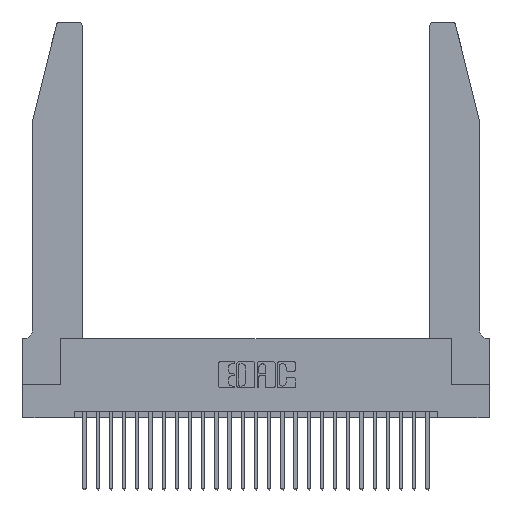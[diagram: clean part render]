
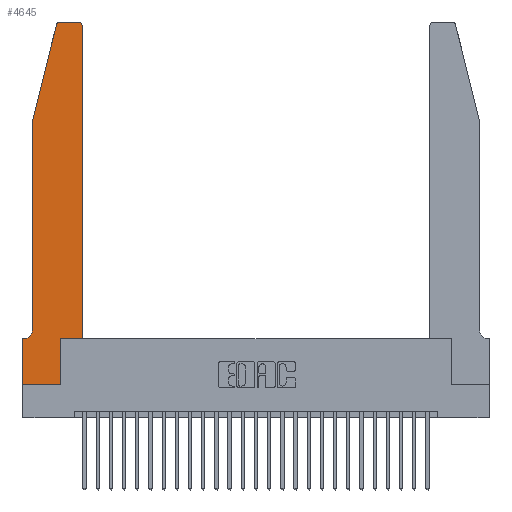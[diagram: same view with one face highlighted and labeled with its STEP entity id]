
A CAD part, top view. The second image highlights one B-rep face of the part: STEP entity #4645.
In plain terms, the highlighted planar face has unit normal (0, 0, 1).
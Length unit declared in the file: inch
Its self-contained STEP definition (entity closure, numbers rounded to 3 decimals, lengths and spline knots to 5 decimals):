
#270 = DIRECTION ( 'NONE',  ( 1., 0., 0. ) ) ;
#932 = DIRECTION ( 'NONE',  ( 1., 0., 0. ) ) ;
#1057 = DIRECTION ( 'NONE',  ( 0., -1., 0. ) ) ;
#1145 = ORIENTED_EDGE ( 'NONE', *, *, #22126, .T. ) ;
#1323 = DIRECTION ( 'NONE',  ( 0., 0., -1. ) ) ;
#1381 = CARTESIAN_POINT ( 'NONE',  ( 0., 0., 0.37 ) ) ;
#1448 = CARTESIAN_POINT ( 'NONE',  ( 0.2605, 2.75, 0.37 ) ) ;
#2068 = VERTEX_POINT ( 'NONE', #8273 ) ;
#2185 = CIRCLE ( 'NONE', #24513, 0.07 ) ;
#3472 = CARTESIAN_POINT ( 'NONE',  ( 0.2865, 0.35, 0.37 ) ) ;
#3636 = EDGE_CURVE ( 'NONE', #10721, #26712, #11440, .T. ) ;
#4051 = EDGE_CURVE ( 'NONE', #22701, #15543, #8329, .T. ) ;
#4174 = VECTOR ( 'NONE', #9013, 39.37008 ) ;
#4192 = CARTESIAN_POINT ( 'NONE',  ( 0.4505, 0.35, 0.37 ) ) ;
#4645 = ADVANCED_FACE ( 'NONE', ( #17044 ), #12396, .T. ) ;
#4649 = EDGE_LOOP ( 'NONE', ( #18988, #1145, #27479, #9173, #19136, #22537, #26817, #24959, #11371, #22296, #23114, #13548 ) ) ;
#5419 = CARTESIAN_POINT ( 'NONE',  ( 0.0755, 2., 0.37 ) ) ;
#5663 = CARTESIAN_POINT ( 'NONE',  ( 0.0755, 0.35, 0.37 ) ) ;
#5740 = CARTESIAN_POINT ( 'NONE',  ( 0.284, 2.72, 0.37 ) ) ;
#5862 = VERTEX_POINT ( 'NONE', #17704 ) ;
#6146 = EDGE_CURVE ( 'NONE', #7760, #11982, #14965, .T. ) ;
#6414 = DIRECTION ( 'NONE',  ( -0.239, -0.971, 0. ) ) ;
#6681 = VERTEX_POINT ( 'NONE', #15907 ) ;
#6736 = VERTEX_POINT ( 'NONE', #22426 ) ;
#7317 = VECTOR ( 'NONE', #6414, 39.37008 ) ;
#7760 = VERTEX_POINT ( 'NONE', #17792 ) ;
#7988 = LINE ( 'NONE', #9923, #18729 ) ;
#7997 = DIRECTION ( 'NONE',  ( 1., 0., 0. ) ) ;
#8273 = CARTESIAN_POINT ( 'NONE',  ( 0.4205, 2.75, 0.37 ) ) ;
#8329 = LINE ( 'NONE', #26907, #23960 ) ;
#8834 = EDGE_CURVE ( 'NONE', #26712, #7760, #22054, .T. ) ;
#9013 = DIRECTION ( 'NONE',  ( 1., 0., 0. ) ) ;
#9173 = ORIENTED_EDGE ( 'NONE', *, *, #4051, .T. ) ;
#9250 = VECTOR ( 'NONE', #18708, 39.37008 ) ;
#9402 = CARTESIAN_POINT ( 'NONE',  ( 0., 0.35, 0.37 ) ) ;
#9532 = CARTESIAN_POINT ( 'NONE',  ( 0., 0., 0.37 ) ) ;
#9923 = CARTESIAN_POINT ( 'NONE',  ( 0.4505, 0.35, 0.37 ) ) ;
#10313 = AXIS2_PLACEMENT_3D ( 'NONE', #14440, #27061, #14529 ) ;
#10721 = VERTEX_POINT ( 'NONE', #9402 ) ;
#11371 = ORIENTED_EDGE ( 'NONE', *, *, #6146, .T. ) ;
#11440 = LINE ( 'NONE', #1381, #22024 ) ;
#11945 = VERTEX_POINT ( 'NONE', #12337 ) ;
#11982 = VERTEX_POINT ( 'NONE', #12436 ) ;
#12146 = DIRECTION ( 'NONE',  ( 0., 1., 0. ) ) ;
#12337 = CARTESIAN_POINT ( 'NONE',  ( 0.25487, 2.72718, 0.37 ) ) ;
#12396 = PLANE ( 'NONE',  #10313 ) ;
#12436 = CARTESIAN_POINT ( 'NONE',  ( 0.2865, 0.35, 0.37 ) ) ;
#12731 = VECTOR ( 'NONE', #18991, 39.37008 ) ;
#13548 = ORIENTED_EDGE ( 'NONE', *, *, #16237, .T. ) ;
#13668 = DIRECTION ( 'NONE',  ( 0., 0., 1. ) ) ;
#14440 = CARTESIAN_POINT ( 'NONE',  ( 0., 0.35, 0.37 ) ) ;
#14529 = DIRECTION ( 'NONE',  ( 1., 0., 0. ) ) ;
#14609 = CARTESIAN_POINT ( 'NONE',  ( 0.0055, 0.42, 0.37 ) ) ;
#14965 = LINE ( 'NONE', #3472, #9250 ) ;
#15543 = VERTEX_POINT ( 'NONE', #18960 ) ;
#15668 = EDGE_CURVE ( 'NONE', #11945, #22701, #23666, .T. ) ;
#15907 = CARTESIAN_POINT ( 'NONE',  ( 0.284, 2.75, 0.37 ) ) ;
#16237 = EDGE_CURVE ( 'NONE', #5862, #2068, #25899, .T. ) ;
#16641 = VERTEX_POINT ( 'NONE', #4192 ) ;
#16737 = DIRECTION ( 'NONE',  ( -1., 0., 0. ) ) ;
#17044 = FACE_OUTER_BOUND ( 'NONE', #4649, .T. ) ;
#17118 = EDGE_CURVE ( 'NONE', #6736, #10721, #27134, .T. ) ;
#17521 = EDGE_CURVE ( 'NONE', #2068, #6681, #24211, .T. ) ;
#17704 = CARTESIAN_POINT ( 'NONE',  ( 0.4505, 2.72, 0.37 ) ) ;
#17792 = CARTESIAN_POINT ( 'NONE',  ( 0.2865, 0., 0.37 ) ) ;
#18708 = DIRECTION ( 'NONE',  ( 0., 1., 0. ) ) ;
#18729 = VECTOR ( 'NONE', #932, 39.37008 ) ;
#18960 = CARTESIAN_POINT ( 'NONE',  ( 0.0755, 0.42, 0.37 ) ) ;
#18988 = ORIENTED_EDGE ( 'NONE', *, *, #17521, .T. ) ;
#18991 = DIRECTION ( 'NONE',  ( -1., 0., 0. ) ) ;
#19136 = ORIENTED_EDGE ( 'NONE', *, *, #22177, .T. ) ;
#20241 = EDGE_CURVE ( 'NONE', #11982, #16641, #7988, .T. ) ;
#20258 = CIRCLE ( 'NONE', #20326, 0.03 ) ;
#20326 = AXIS2_PLACEMENT_3D ( 'NONE', #5740, #20801, #7997 ) ;
#20412 = AXIS2_PLACEMENT_3D ( 'NONE', #26217, #13668, #270 ) ;
#20801 = DIRECTION ( 'NONE',  ( 0., 0., 1. ) ) ;
#21046 = DIRECTION ( 'NONE',  ( 0., -1., 0. ) ) ;
#21622 = VECTOR ( 'NONE', #24896, 39.37008 ) ;
#22024 = VECTOR ( 'NONE', #21046, 39.37008 ) ;
#22054 = LINE ( 'NONE', #23857, #4174 ) ;
#22126 = EDGE_CURVE ( 'NONE', #6681, #11945, #20258, .T. ) ;
#22177 = EDGE_CURVE ( 'NONE', #15543, #6736, #2185, .T. ) ;
#22296 = ORIENTED_EDGE ( 'NONE', *, *, #20241, .T. ) ;
#22426 = CARTESIAN_POINT ( 'NONE',  ( 0.0055, 0.35, 0.37 ) ) ;
#22537 = ORIENTED_EDGE ( 'NONE', *, *, #17118, .T. ) ;
#22648 = CARTESIAN_POINT ( 'NONE',  ( 0.4505, 0.35, 0.37 ) ) ;
#22689 = LINE ( 'NONE', #22648, #27566 ) ;
#22701 = VERTEX_POINT ( 'NONE', #5419 ) ;
#23114 = ORIENTED_EDGE ( 'NONE', *, *, #27883, .T. ) ;
#23666 = LINE ( 'NONE', #25600, #7317 ) ;
#23857 = CARTESIAN_POINT ( 'NONE',  ( 0., 0., 0.37 ) ) ;
#23960 = VECTOR ( 'NONE', #1057, 39.37008 ) ;
#24211 = LINE ( 'NONE', #1448, #12731 ) ;
#24513 = AXIS2_PLACEMENT_3D ( 'NONE', #14609, #1323, #16737 ) ;
#24896 = DIRECTION ( 'NONE',  ( -1., 0., 0. ) ) ;
#24959 = ORIENTED_EDGE ( 'NONE', *, *, #8834, .T. ) ;
#25600 = CARTESIAN_POINT ( 'NONE',  ( 0.0755, 2., 0.37 ) ) ;
#25899 = CIRCLE ( 'NONE', #20412, 0.03 ) ;
#26217 = CARTESIAN_POINT ( 'NONE',  ( 0.4205, 2.72, 0.37 ) ) ;
#26712 = VERTEX_POINT ( 'NONE', #9532 ) ;
#26817 = ORIENTED_EDGE ( 'NONE', *, *, #3636, .T. ) ;
#26907 = CARTESIAN_POINT ( 'NONE',  ( 0.0755, 2., 0.37 ) ) ;
#27061 = DIRECTION ( 'NONE',  ( 0., 0., 1. ) ) ;
#27134 = LINE ( 'NONE', #5663, #21622 ) ;
#27479 = ORIENTED_EDGE ( 'NONE', *, *, #15668, .T. ) ;
#27566 = VECTOR ( 'NONE', #12146, 39.37008 ) ;
#27883 = EDGE_CURVE ( 'NONE', #16641, #5862, #22689, .T. ) ;
